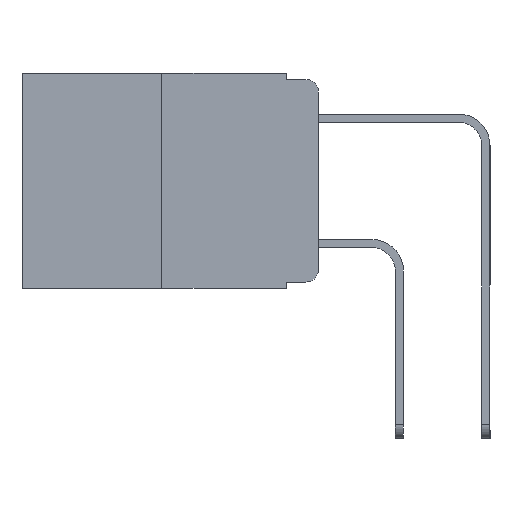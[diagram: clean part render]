
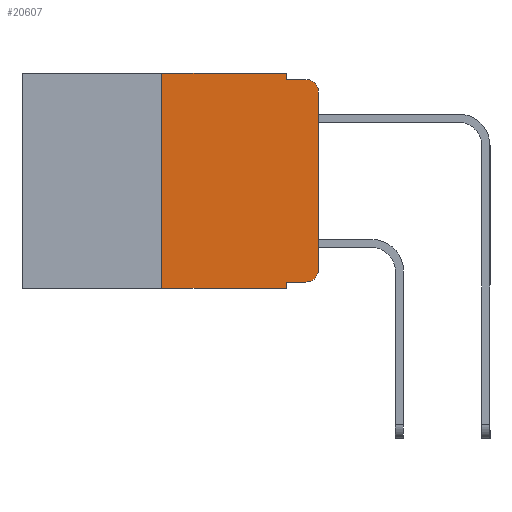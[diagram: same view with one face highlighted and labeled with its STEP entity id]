
A CAD part, left-side view. The second image highlights one B-rep face of the part: STEP entity #20607.
In plain terms, the highlighted planar face has unit normal (-1, 0, 0).
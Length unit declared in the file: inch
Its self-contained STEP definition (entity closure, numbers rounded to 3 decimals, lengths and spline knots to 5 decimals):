
#83 = VECTOR ( 'NONE', #16356, 39.37008 ) ;
#135 = AXIS2_PLACEMENT_3D ( 'NONE', #21623, #10821, #23413 ) ;
#139 = VERTEX_POINT ( 'NONE', #2531 ) ;
#339 = CARTESIAN_POINT ( 'NONE',  ( 0., 0.02, -0.333 ) ) ;
#424 = CARTESIAN_POINT ( 'NONE',  ( 0., 0., 0. ) ) ;
#620 = CARTESIAN_POINT ( 'NONE',  ( 0., 0.051, -0.01 ) ) ;
#997 = LINE ( 'NONE', #6804, #9844 ) ;
#1149 = VERTEX_POINT ( 'NONE', #339 ) ;
#1596 = DIRECTION ( 'NONE',  ( 0., 0., -1. ) ) ;
#1873 = ORIENTED_EDGE ( 'NONE', *, *, #7989, .F. ) ;
#2340 = VECTOR ( 'NONE', #7788, 39.37008 ) ;
#2531 = CARTESIAN_POINT ( 'NONE',  ( 0., 0.051, -0.333 ) ) ;
#2551 = DIRECTION ( 'NONE',  ( 0., -1., 0. ) ) ;
#2578 = VECTOR ( 'NONE', #2551, 39.37008 ) ;
#2806 = LINE ( 'NONE', #5474, #12723 ) ;
#3083 = EDGE_CURVE ( 'NONE', #7157, #21695, #17101, .T. ) ;
#3321 = VERTEX_POINT ( 'NONE', #5091 ) ;
#4266 = ORIENTED_EDGE ( 'NONE', *, *, #17746, .T. ) ;
#4292 = CIRCLE ( 'NONE', #5886, 0.02 ) ;
#4553 = ORIENTED_EDGE ( 'NONE', *, *, #17183, .T. ) ;
#5091 = CARTESIAN_POINT ( 'NONE',  ( 0., 0., -0.313 ) ) ;
#5193 = LINE ( 'NONE', #23481, #83 ) ;
#5333 = CARTESIAN_POINT ( 'NONE',  ( 0., 0.473, -0.343 ) ) ;
#5474 = CARTESIAN_POINT ( 'NONE',  ( 0., 0.051, 0. ) ) ;
#5752 = ORIENTED_EDGE ( 'NONE', *, *, #18487, .F. ) ;
#5790 = CARTESIAN_POINT ( 'NONE',  ( 0., 0.02, -0.01 ) ) ;
#5842 = VERTEX_POINT ( 'NONE', #15416 ) ;
#5886 = AXIS2_PLACEMENT_3D ( 'NONE', #21020, #10191, #22837 ) ;
#6174 = DIRECTION ( 'NONE',  ( 0., 0., 1. ) ) ;
#6804 = CARTESIAN_POINT ( 'NONE',  ( 0., 0.473, 0. ) ) ;
#7157 = VERTEX_POINT ( 'NONE', #22576 ) ;
#7166 = VERTEX_POINT ( 'NONE', #22652 ) ;
#7246 = PLANE ( 'NONE',  #13170 ) ;
#7382 = CARTESIAN_POINT ( 'NONE',  ( 0., 0.051, 0. ) ) ;
#7610 = LINE ( 'NONE', #620, #2578 ) ;
#7788 = DIRECTION ( 'NONE',  ( 0., -1., 0. ) ) ;
#7989 = EDGE_CURVE ( 'NONE', #7157, #5842, #8135, .T. ) ;
#8135 = LINE ( 'NONE', #11919, #16134 ) ;
#8932 = CARTESIAN_POINT ( 'NONE',  ( 0., 0.051, -0.343 ) ) ;
#9117 = VECTOR ( 'NONE', #18739, 39.37008 ) ;
#9530 = EDGE_CURVE ( 'NONE', #1149, #3321, #22779, .T. ) ;
#9844 = VECTOR ( 'NONE', #17731, 39.37008 ) ;
#10191 = DIRECTION ( 'NONE',  ( -1., 0., 0. ) ) ;
#10821 = DIRECTION ( 'NONE',  ( -1., 0., 0. ) ) ;
#11919 = CARTESIAN_POINT ( 'NONE',  ( 0., 0.25, 0. ) ) ;
#11936 = EDGE_CURVE ( 'NONE', #5842, #23353, #997, .T. ) ;
#12723 = VECTOR ( 'NONE', #18246, 39.37008 ) ;
#12733 = CARTESIAN_POINT ( 'NONE',  ( 0., 0.473, 0. ) ) ;
#12813 = DIRECTION ( 'NONE',  ( 1., 0., 0. ) ) ;
#13170 = AXIS2_PLACEMENT_3D ( 'NONE', #12733, #12813, #1596 ) ;
#14203 = VECTOR ( 'NONE', #6174, 39.37008 ) ;
#14679 = VERTEX_POINT ( 'NONE', #5790 ) ;
#15416 = CARTESIAN_POINT ( 'NONE',  ( 0., 0.25, 0. ) ) ;
#15524 = ORIENTED_EDGE ( 'NONE', *, *, #19989, .F. ) ;
#15565 = DIRECTION ( 'NONE',  ( 0., 0., 1. ) ) ;
#15868 = VERTEX_POINT ( 'NONE', #21987 ) ;
#16134 = VECTOR ( 'NONE', #15565, 39.37008 ) ;
#16356 = DIRECTION ( 'NONE',  ( 0., 0., -1. ) ) ;
#17101 = LINE ( 'NONE', #5333, #2340 ) ;
#17183 = EDGE_CURVE ( 'NONE', #3321, #7166, #18939, .T. ) ;
#17731 = DIRECTION ( 'NONE',  ( 0., -1., 0. ) ) ;
#17746 = EDGE_CURVE ( 'NONE', #139, #1149, #18720, .T. ) ;
#18246 = DIRECTION ( 'NONE',  ( 0., 0., -1. ) ) ;
#18463 = EDGE_LOOP ( 'NONE', ( #4553, #19743, #5752, #15524, #20852, #1873, #22001, #23123, #4266, #19456 ) ) ;
#18487 = EDGE_CURVE ( 'NONE', #15868, #14679, #7610, .T. ) ;
#18720 = LINE ( 'NONE', #18817, #9117 ) ;
#18739 = DIRECTION ( 'NONE',  ( 0., -1., 0. ) ) ;
#18817 = CARTESIAN_POINT ( 'NONE',  ( 0., 0.051, -0.333 ) ) ;
#18939 = LINE ( 'NONE', #424, #14203 ) ;
#19456 = ORIENTED_EDGE ( 'NONE', *, *, #9530, .T. ) ;
#19716 = EDGE_CURVE ( 'NONE', #7166, #14679, #4292, .T. ) ;
#19743 = ORIENTED_EDGE ( 'NONE', *, *, #19716, .T. ) ;
#19989 = EDGE_CURVE ( 'NONE', #23353, #15868, #2806, .T. ) ;
#20589 = EDGE_CURVE ( 'NONE', #139, #21695, #5193, .T. ) ;
#20607 = ADVANCED_FACE ( 'NONE', ( #23398 ), #7246, .F. ) ;
#20852 = ORIENTED_EDGE ( 'NONE', *, *, #11936, .F. ) ;
#21020 = CARTESIAN_POINT ( 'NONE',  ( 0., 0.02, -0.03 ) ) ;
#21623 = CARTESIAN_POINT ( 'NONE',  ( 0., 0.02, -0.313 ) ) ;
#21695 = VERTEX_POINT ( 'NONE', #8932 ) ;
#21987 = CARTESIAN_POINT ( 'NONE',  ( 0., 0.051, -0.01 ) ) ;
#22001 = ORIENTED_EDGE ( 'NONE', *, *, #3083, .T. ) ;
#22576 = CARTESIAN_POINT ( 'NONE',  ( 0., 0.25, -0.343 ) ) ;
#22652 = CARTESIAN_POINT ( 'NONE',  ( 0., 0., -0.03 ) ) ;
#22779 = CIRCLE ( 'NONE', #135, 0.02 ) ;
#22837 = DIRECTION ( 'NONE',  ( 0., 0., -1. ) ) ;
#23123 = ORIENTED_EDGE ( 'NONE', *, *, #20589, .F. ) ;
#23353 = VERTEX_POINT ( 'NONE', #7382 ) ;
#23398 = FACE_OUTER_BOUND ( 'NONE', #18463, .T. ) ;
#23413 = DIRECTION ( 'NONE',  ( 0., 0., -1. ) ) ;
#23481 = CARTESIAN_POINT ( 'NONE',  ( 0., 0.051, 0. ) ) ;
